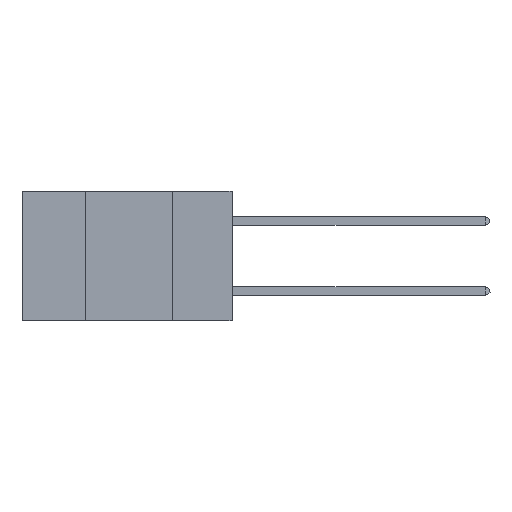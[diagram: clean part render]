
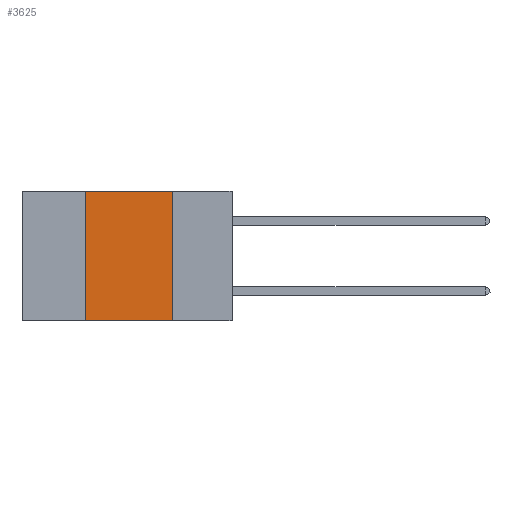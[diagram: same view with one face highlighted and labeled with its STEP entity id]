
A CAD part, left-side view. The second image highlights one B-rep face of the part: STEP entity #3625.
In plain terms, the highlighted planar face has unit normal (-1, 0, 0).
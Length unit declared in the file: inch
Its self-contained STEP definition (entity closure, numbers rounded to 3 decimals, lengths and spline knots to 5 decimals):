
#96 = VERTEX_POINT ( 'NONE', #6675 ) ;
#330 = EDGE_CURVE ( 'NONE', #6181, #96, #19807, .T. ) ;
#744 = CARTESIAN_POINT ( 'NONE',  ( 0., 0.42, -0.37 ) ) ;
#1003 = VECTOR ( 'NONE', #14934, 39.37008 ) ;
#1830 = DIRECTION ( 'NONE',  ( 1., 0., 0. ) ) ;
#3272 = ORIENTED_EDGE ( 'NONE', *, *, #330, .F. ) ;
#3625 = ADVANCED_FACE ( 'NONE', ( #13522 ), #6390, .F. ) ;
#4140 = EDGE_CURVE ( 'NONE', #27002, #19822, #13813, .T. ) ;
#4202 = VECTOR ( 'NONE', #29173, 39.37008 ) ;
#5031 = CARTESIAN_POINT ( 'NONE',  ( 0., 0.42, 0. ) ) ;
#6181 = VERTEX_POINT ( 'NONE', #744 ) ;
#6390 = PLANE ( 'NONE',  #12619 ) ;
#6675 = CARTESIAN_POINT ( 'NONE',  ( 0., 0.42, 0. ) ) ;
#9612 = ORIENTED_EDGE ( 'NONE', *, *, #26367, .T. ) ;
#10425 = EDGE_LOOP ( 'NONE', ( #20614, #24343, #3272, #9612 ) ) ;
#10520 = LINE ( 'NONE', #20425, #30626 ) ;
#11372 = DIRECTION ( 'NONE',  ( 0., 0., -1. ) ) ;
#11993 = CARTESIAN_POINT ( 'NONE',  ( 0., 0.6, 0. ) ) ;
#12619 = AXIS2_PLACEMENT_3D ( 'NONE', #24030, #1830, #20990 ) ;
#13522 = FACE_OUTER_BOUND ( 'NONE', #10425, .T. ) ;
#13813 = LINE ( 'NONE', #23685, #27176 ) ;
#14934 = DIRECTION ( 'NONE',  ( 0., 0., 1. ) ) ;
#18540 = CARTESIAN_POINT ( 'NONE',  ( 0., 0.17, -0.37 ) ) ;
#18858 = DIRECTION ( 'NONE',  ( 0., -1., 0. ) ) ;
#19807 = LINE ( 'NONE', #5031, #1003 ) ;
#19822 = VERTEX_POINT ( 'NONE', #18540 ) ;
#20425 = CARTESIAN_POINT ( 'NONE',  ( 0., 0.6, -0.37 ) ) ;
#20614 = ORIENTED_EDGE ( 'NONE', *, *, #4140, .F. ) ;
#20990 = DIRECTION ( 'NONE',  ( 0., 0., -1. ) ) ;
#23685 = CARTESIAN_POINT ( 'NONE',  ( 0., 0.17, 0. ) ) ;
#24030 = CARTESIAN_POINT ( 'NONE',  ( 0., 0.6, 0. ) ) ;
#24157 = EDGE_CURVE ( 'NONE', #96, #27002, #29646, .T. ) ;
#24343 = ORIENTED_EDGE ( 'NONE', *, *, #24157, .F. ) ;
#26367 = EDGE_CURVE ( 'NONE', #6181, #19822, #10520, .T. ) ;
#27002 = VERTEX_POINT ( 'NONE', #31210 ) ;
#27176 = VECTOR ( 'NONE', #11372, 39.37008 ) ;
#29173 = DIRECTION ( 'NONE',  ( 0., -1., 0. ) ) ;
#29646 = LINE ( 'NONE', #11993, #4202 ) ;
#30626 = VECTOR ( 'NONE', #18858, 39.37008 ) ;
#31210 = CARTESIAN_POINT ( 'NONE',  ( 0., 0.17, 0. ) ) ;
